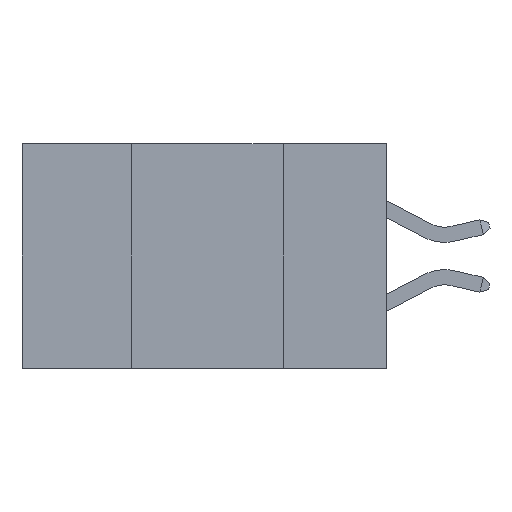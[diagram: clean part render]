
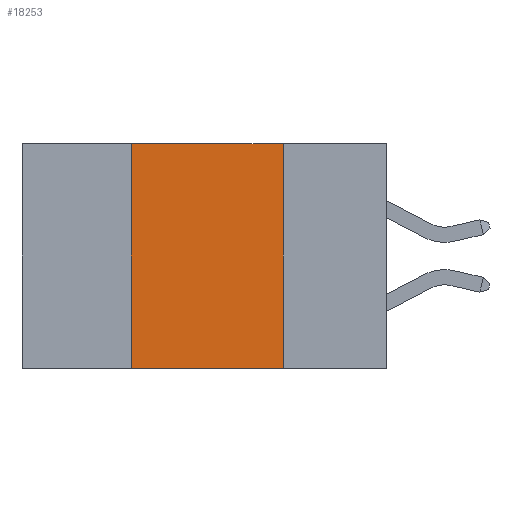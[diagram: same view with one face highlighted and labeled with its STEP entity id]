
A CAD part, left-side view. The second image highlights one B-rep face of the part: STEP entity #18253.
In plain terms, the highlighted planar face has unit normal (-1, 0, 0).
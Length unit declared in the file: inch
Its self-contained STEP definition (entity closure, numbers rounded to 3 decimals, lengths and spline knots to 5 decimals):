
#944 = EDGE_LOOP ( 'NONE', ( #9357, #2051, #3378, #15011 ) ) ;
#1635 = DIRECTION ( 'NONE',  ( 0., 0., 1. ) ) ;
#2051 = ORIENTED_EDGE ( 'NONE', *, *, #3758, .F. ) ;
#2339 = CARTESIAN_POINT ( 'NONE',  ( 0., 0.42, -0.37 ) ) ;
#2646 = CARTESIAN_POINT ( 'NONE',  ( 0., 0.6, 0. ) ) ;
#3207 = VERTEX_POINT ( 'NONE', #17005 ) ;
#3378 = ORIENTED_EDGE ( 'NONE', *, *, #21328, .F. ) ;
#3758 = EDGE_CURVE ( 'NONE', #20228, #3207, #13742, .T. ) ;
#4294 = CARTESIAN_POINT ( 'NONE',  ( 0., 0.17, -0.37 ) ) ;
#4587 = CARTESIAN_POINT ( 'NONE',  ( 0., 0.17, 0. ) ) ;
#4661 = VECTOR ( 'NONE', #18940, 39.37008 ) ;
#4844 = CARTESIAN_POINT ( 'NONE',  ( 0., 0.6, -0.37 ) ) ;
#5171 = LINE ( 'NONE', #25536, #15250 ) ;
#6671 = DIRECTION ( 'NONE',  ( 1., 0., 0. ) ) ;
#8343 = VECTOR ( 'NONE', #16289, 39.37008 ) ;
#9357 = ORIENTED_EDGE ( 'NONE', *, *, #12715, .F. ) ;
#10559 = CARTESIAN_POINT ( 'NONE',  ( 0., 0.42, 0. ) ) ;
#10894 = EDGE_CURVE ( 'NONE', #18827, #18802, #20096, .T. ) ;
#12715 = EDGE_CURVE ( 'NONE', #3207, #18802, #20615, .T. ) ;
#13742 = LINE ( 'NONE', #16324, #8343 ) ;
#14713 = PLANE ( 'NONE',  #23877 ) ;
#15011 = ORIENTED_EDGE ( 'NONE', *, *, #10894, .T. ) ;
#15250 = VECTOR ( 'NONE', #1635, 39.37008 ) ;
#16289 = DIRECTION ( 'NONE',  ( 0., -1., 0. ) ) ;
#16324 = CARTESIAN_POINT ( 'NONE',  ( 0., 0.6, 0. ) ) ;
#17005 = CARTESIAN_POINT ( 'NONE',  ( 0., 0.17, 0. ) ) ;
#18253 = ADVANCED_FACE ( 'NONE', ( #21363 ), #14713, .F. ) ;
#18802 = VERTEX_POINT ( 'NONE', #4294 ) ;
#18827 = VERTEX_POINT ( 'NONE', #2339 ) ;
#18940 = DIRECTION ( 'NONE',  ( 0., -1., 0. ) ) ;
#20004 = VECTOR ( 'NONE', #20682, 39.37008 ) ;
#20096 = LINE ( 'NONE', #4844, #4661 ) ;
#20228 = VERTEX_POINT ( 'NONE', #10559 ) ;
#20615 = LINE ( 'NONE', #4587, #20004 ) ;
#20682 = DIRECTION ( 'NONE',  ( 0., 0., -1. ) ) ;
#20753 = DIRECTION ( 'NONE',  ( 0., 0., -1. ) ) ;
#21328 = EDGE_CURVE ( 'NONE', #18827, #20228, #5171, .T. ) ;
#21363 = FACE_OUTER_BOUND ( 'NONE', #944, .T. ) ;
#23877 = AXIS2_PLACEMENT_3D ( 'NONE', #2646, #6671, #20753 ) ;
#25536 = CARTESIAN_POINT ( 'NONE',  ( 0., 0.42, 0. ) ) ;
